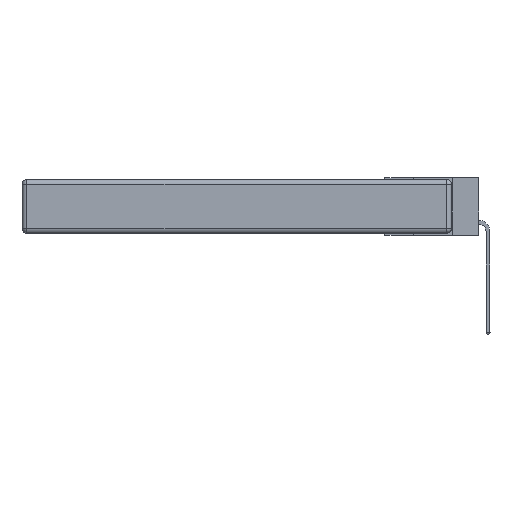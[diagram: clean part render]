
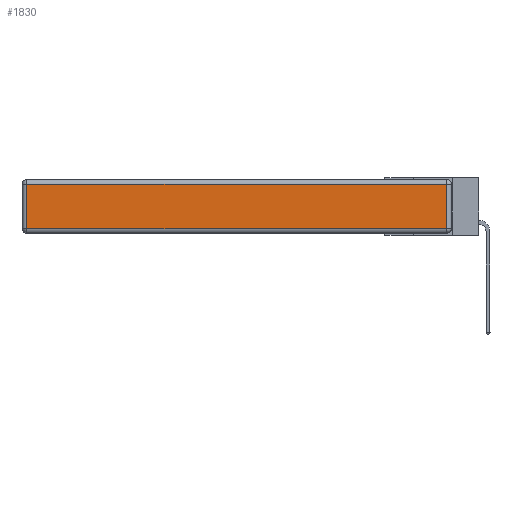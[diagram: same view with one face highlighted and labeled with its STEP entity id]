
A CAD part, left-side view. The second image highlights one B-rep face of the part: STEP entity #1830.
In plain terms, the highlighted planar face has unit normal (-1, 0, 0).
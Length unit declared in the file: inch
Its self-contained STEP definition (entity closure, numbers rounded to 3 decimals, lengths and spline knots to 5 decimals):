
#66 = FACE_OUTER_BOUND ( 'NONE', #8829, .T. ) ;
#164 = DIRECTION ( 'NONE',  ( 0., -1., 0. ) ) ;
#605 = EDGE_CURVE ( 'NONE', #3436, #3511, #6139, .T. ) ;
#846 = VECTOR ( 'NONE', #4251, 39.37008 ) ;
#994 = ORIENTED_EDGE ( 'NONE', *, *, #605, .T. ) ;
#1830 = ADVANCED_FACE ( 'NONE', ( #66 ), #12288, .T. ) ;
#2015 = CARTESIAN_POINT ( 'NONE',  ( 0., 0.03, -0.343 ) ) ;
#2194 = EDGE_CURVE ( 'NONE', #3511, #7138, #9238, .T. ) ;
#2990 = DIRECTION ( 'NONE',  ( 0., 0., 1. ) ) ;
#3436 = VERTEX_POINT ( 'NONE', #12483 ) ;
#3511 = VERTEX_POINT ( 'NONE', #14166 ) ;
#4062 = CARTESIAN_POINT ( 'NONE',  ( 0., 2.75, -0.03 ) ) ;
#4251 = DIRECTION ( 'NONE',  ( 0., 0., 1. ) ) ;
#4647 = VECTOR ( 'NONE', #14807, 39.37008 ) ;
#5587 = EDGE_CURVE ( 'NONE', #7138, #9604, #6129, .T. ) ;
#6129 = LINE ( 'NONE', #2015, #846 ) ;
#6139 = LINE ( 'NONE', #14522, #9103 ) ;
#6339 = ORIENTED_EDGE ( 'NONE', *, *, #5587, .T. ) ;
#7138 = VERTEX_POINT ( 'NONE', #7620 ) ;
#7229 = ORIENTED_EDGE ( 'NONE', *, *, #10819, .T. ) ;
#7620 = CARTESIAN_POINT ( 'NONE',  ( 0., 0.03, -0.313 ) ) ;
#8829 = EDGE_LOOP ( 'NONE', ( #10980, #6339, #7229, #994 ) ) ;
#9033 = AXIS2_PLACEMENT_3D ( 'NONE', #10030, #11146, #2990 ) ;
#9103 = VECTOR ( 'NONE', #14615, 39.37008 ) ;
#9238 = LINE ( 'NONE', #9456, #9419 ) ;
#9419 = VECTOR ( 'NONE', #164, 39.37008 ) ;
#9456 = CARTESIAN_POINT ( 'NONE',  ( 0., 0., -0.313 ) ) ;
#9604 = VERTEX_POINT ( 'NONE', #11000 ) ;
#10014 = LINE ( 'NONE', #4062, #4647 ) ;
#10030 = CARTESIAN_POINT ( 'NONE',  ( 0., 0., -0.343 ) ) ;
#10819 = EDGE_CURVE ( 'NONE', #9604, #3436, #10014, .T. ) ;
#10980 = ORIENTED_EDGE ( 'NONE', *, *, #2194, .T. ) ;
#11000 = CARTESIAN_POINT ( 'NONE',  ( 0., 0.03, -0.03 ) ) ;
#11146 = DIRECTION ( 'NONE',  ( -1., 0., 0. ) ) ;
#12288 = PLANE ( 'NONE',  #9033 ) ;
#12483 = CARTESIAN_POINT ( 'NONE',  ( 0., 2.72, -0.03 ) ) ;
#14166 = CARTESIAN_POINT ( 'NONE',  ( 0., 2.72, -0.313 ) ) ;
#14522 = CARTESIAN_POINT ( 'NONE',  ( 0., 2.72, -0.343 ) ) ;
#14615 = DIRECTION ( 'NONE',  ( 0., 0., -1. ) ) ;
#14807 = DIRECTION ( 'NONE',  ( 0., 1., 0. ) ) ;
